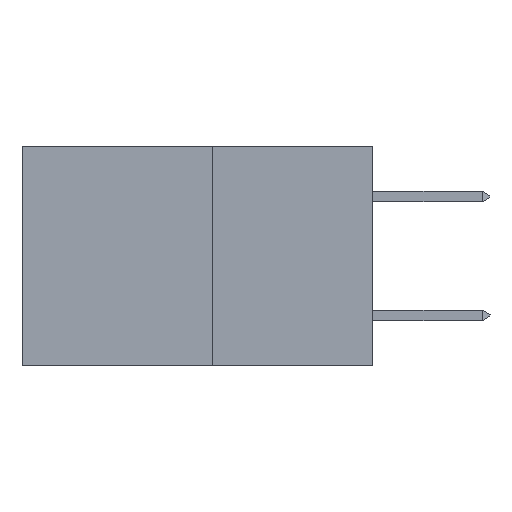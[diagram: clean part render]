
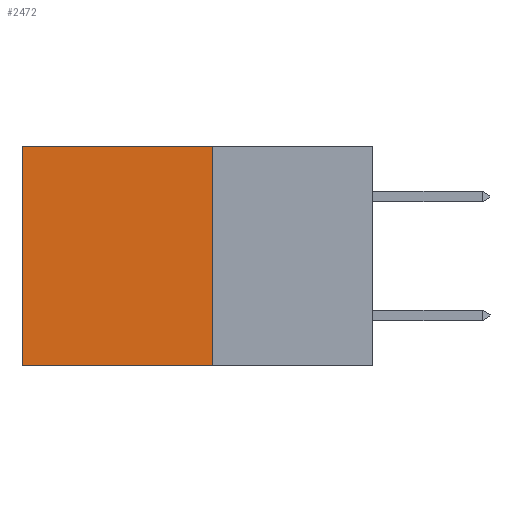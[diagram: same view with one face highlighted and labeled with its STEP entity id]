
A CAD part, left-side view. The second image highlights one B-rep face of the part: STEP entity #2472.
In plain terms, the highlighted planar face has unit normal (-1, 0, 0).
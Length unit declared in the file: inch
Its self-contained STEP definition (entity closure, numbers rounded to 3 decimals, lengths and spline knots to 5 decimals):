
#933 = AXIS2_PLACEMENT_3D ( 'NONE', #8213, #8143, #8184 ) ;
#1154 = ORIENTED_EDGE ( 'NONE', *, *, #2279, .T. ) ;
#1338 = CARTESIAN_POINT ( 'NONE',  ( 0.277, 0.27, -0.37 ) ) ;
#2279 = EDGE_CURVE ( 'NONE', #6596, #13292, #4308, .T. ) ;
#2467 = DIRECTION ( 'NONE',  ( 0., 0., -1. ) ) ;
#2472 = ADVANCED_FACE ( 'NONE', ( #9101 ), #8337, .F. ) ;
#2575 = CARTESIAN_POINT ( 'NONE',  ( 0.277, 0.59, -0.37 ) ) ;
#3884 = VECTOR ( 'NONE', #4706, 39.37008 ) ;
#4242 = EDGE_CURVE ( 'NONE', #6596, #7436, #13439, .T. ) ;
#4308 = LINE ( 'NONE', #7101, #10034 ) ;
#4684 = CARTESIAN_POINT ( 'NONE',  ( 0.277, 0.27, -0.37 ) ) ;
#4706 = DIRECTION ( 'NONE',  ( 0., 0., -1. ) ) ;
#4809 = CARTESIAN_POINT ( 'NONE',  ( 0.277, 0.27, 0. ) ) ;
#5742 = EDGE_CURVE ( 'NONE', #13292, #11151, #5975, .T. ) ;
#5975 = LINE ( 'NONE', #2575, #11377 ) ;
#6397 = ORIENTED_EDGE ( 'NONE', *, *, #4242, .F. ) ;
#6596 = VERTEX_POINT ( 'NONE', #4809 ) ;
#7101 = CARTESIAN_POINT ( 'NONE',  ( 0.277, 0.27, 0. ) ) ;
#7131 = VECTOR ( 'NONE', #10413, 39.37008 ) ;
#7436 = VERTEX_POINT ( 'NONE', #1338 ) ;
#8143 = DIRECTION ( 'NONE',  ( 1., 0., 0. ) ) ;
#8184 = DIRECTION ( 'NONE',  ( 0., 0., -1. ) ) ;
#8189 = ORIENTED_EDGE ( 'NONE', *, *, #5742, .T. ) ;
#8213 = CARTESIAN_POINT ( 'NONE',  ( 0.277, 0.27, -0.37 ) ) ;
#8337 = PLANE ( 'NONE',  #933 ) ;
#8638 = EDGE_CURVE ( 'NONE', #7436, #11151, #13323, .T. ) ;
#8907 = ORIENTED_EDGE ( 'NONE', *, *, #8638, .F. ) ;
#9101 = FACE_OUTER_BOUND ( 'NONE', #10032, .T. ) ;
#9250 = CARTESIAN_POINT ( 'NONE',  ( 0.277, 0.27, -0.37 ) ) ;
#10032 = EDGE_LOOP ( 'NONE', ( #8189, #8907, #6397, #1154 ) ) ;
#10034 = VECTOR ( 'NONE', #13352, 39.37008 ) ;
#10413 = DIRECTION ( 'NONE',  ( 0., 1., 0. ) ) ;
#10596 = CARTESIAN_POINT ( 'NONE',  ( 0.277, 0.59, -0.37 ) ) ;
#11151 = VERTEX_POINT ( 'NONE', #10596 ) ;
#11377 = VECTOR ( 'NONE', #2467, 39.37008 ) ;
#13292 = VERTEX_POINT ( 'NONE', #13537 ) ;
#13323 = LINE ( 'NONE', #9250, #7131 ) ;
#13352 = DIRECTION ( 'NONE',  ( 0., 1., 0. ) ) ;
#13439 = LINE ( 'NONE', #4684, #3884 ) ;
#13537 = CARTESIAN_POINT ( 'NONE',  ( 0.277, 0.59, 0. ) ) ;
